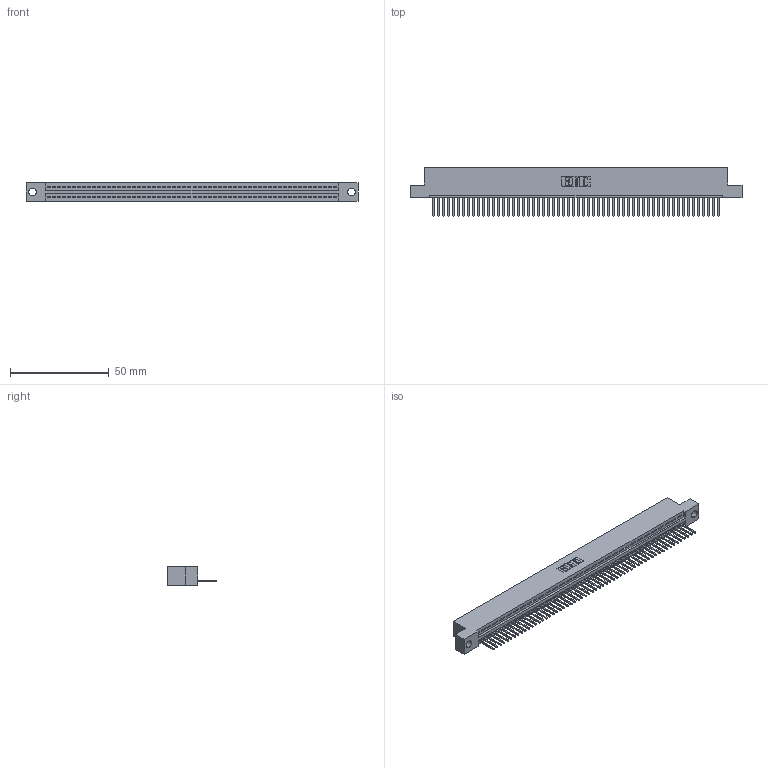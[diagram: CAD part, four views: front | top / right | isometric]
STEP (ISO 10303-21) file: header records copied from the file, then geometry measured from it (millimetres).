
FILE_DESCRIPTION (( 'STEP AP203' ), '1' );
FILE_NAME ('345-058-523-104.STEP', '2021-05-28T15:42:22', ( '' ), ( '' ), 'SwSTEP 2.0', 'SolidWorks 2020', '' );
FILE_SCHEMA (( 'CONFIG_CONTROL_DESIGN' ));
Length unit declared in the file: inch
Products named in the file (3): 345 Part_Flush Mounting Lugs - 0.156 Dia-TI; 345-292-001_345-293-123; 345-058-523-104
Assembly tree (59 placements, depth 2):
  345-058-523-104
    345 Part_Flush Mounting Lugs - 0.156 Dia-TI
    345-292-001_345-293-123  x58
Bounding box: 168.53 x 24.82 x 9.4 mm (x, y, z)
Volume: 16009.7 mm3; surface area: 21398.6 mm2
Topology: 59 solids, 59 shells, 3504 faces, 10585 edges, 6978 vertices
Faces by surface type: plane 2414, cylinder 1090
Entity records: 41935 total; most frequent: CARTESIAN_POINT 7272, ORIENTED_EDGE 7262, DIRECTION 6327, EDGE_CURVE 3631, VECTOR 3267, LINE 3267, VERTEX_POINT 2418, AXIS2_PLACEMENT_3D 1530
